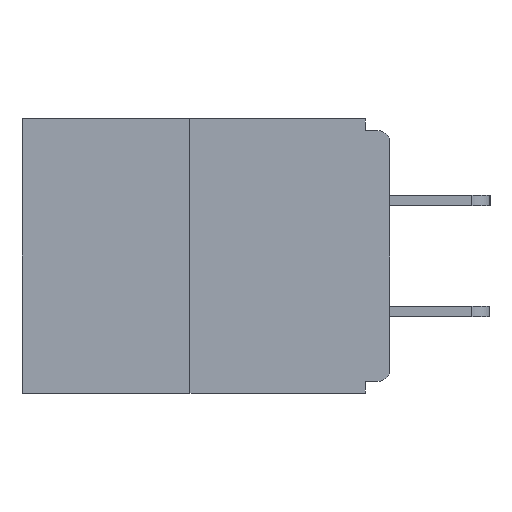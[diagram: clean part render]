
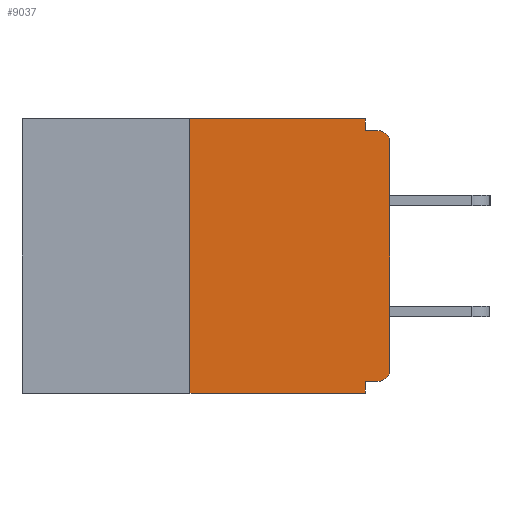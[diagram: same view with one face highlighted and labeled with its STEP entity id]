
A CAD part, left-side view. The second image highlights one B-rep face of the part: STEP entity #9037.
In plain terms, the highlighted planar face has unit normal (-1, 0, 0).
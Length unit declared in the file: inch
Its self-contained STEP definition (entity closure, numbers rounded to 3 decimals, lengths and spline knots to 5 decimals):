
#4 = ORIENTED_EDGE ( 'NONE', *, *, #11150, .F. ) ;
#123 = EDGE_LOOP ( 'NONE', ( #939, #2051, #2293, #3961, #8001, #12111, #1649, #12797, #4116, #4 ) ) ;
#710 = VERTEX_POINT ( 'NONE', #12947 ) ;
#714 = CARTESIAN_POINT ( 'NONE',  ( 0., 0., -0.313 ) ) ;
#939 = ORIENTED_EDGE ( 'NONE', *, *, #2842, .F. ) ;
#1029 = CARTESIAN_POINT ( 'NONE',  ( 0., 0.46, 0. ) ) ;
#1086 = VECTOR ( 'NONE', #10033, 39.37008 ) ;
#1126 = CARTESIAN_POINT ( 'NONE',  ( 0., 0., -0.015 ) ) ;
#1252 = AXIS2_PLACEMENT_3D ( 'NONE', #8009, #3715, #13495 ) ;
#1649 = ORIENTED_EDGE ( 'NONE', *, *, #4518, .T. ) ;
#1682 = DIRECTION ( 'NONE',  ( 0., -1., 0. ) ) ;
#2051 = ORIENTED_EDGE ( 'NONE', *, *, #3846, .F. ) ;
#2113 = DIRECTION ( 'NONE',  ( 0., 0., -1. ) ) ;
#2199 = CARTESIAN_POINT ( 'NONE',  ( 0., 0.25, -0.343 ) ) ;
#2293 = ORIENTED_EDGE ( 'NONE', *, *, #7342, .T. ) ;
#2337 = CARTESIAN_POINT ( 'NONE',  ( 0., 0., -0.328 ) ) ;
#2506 = EDGE_CURVE ( 'NONE', #710, #9121, #10953, .T. ) ;
#2724 = DIRECTION ( 'NONE',  ( 0., 0., -1. ) ) ;
#2842 = EDGE_CURVE ( 'NONE', #11272, #7863, #7453, .T. ) ;
#2844 = DIRECTION ( 'NONE',  ( 0., 0., -1. ) ) ;
#3368 = AXIS2_PLACEMENT_3D ( 'NONE', #10597, #12603, #2844 ) ;
#3414 = CARTESIAN_POINT ( 'NONE',  ( 0., 0., 0. ) ) ;
#3503 = CARTESIAN_POINT ( 'NONE',  ( 0., 0.031, -0.328 ) ) ;
#3594 = EDGE_CURVE ( 'NONE', #7146, #11000, #7403, .T. ) ;
#3715 = DIRECTION ( 'NONE',  ( -1., 0., 0. ) ) ;
#3846 = EDGE_CURVE ( 'NONE', #4513, #11272, #9178, .T. ) ;
#3870 = CARTESIAN_POINT ( 'NONE',  ( 0., 0.015, -0.015 ) ) ;
#3961 = ORIENTED_EDGE ( 'NONE', *, *, #8434, .F. ) ;
#4116 = ORIENTED_EDGE ( 'NONE', *, *, #2506, .F. ) ;
#4135 = DIRECTION ( 'NONE',  ( 0., -1., 0. ) ) ;
#4455 = VECTOR ( 'NONE', #14008, 39.37008 ) ;
#4478 = LINE ( 'NONE', #2337, #6018 ) ;
#4513 = VERTEX_POINT ( 'NONE', #2199 ) ;
#4518 = EDGE_CURVE ( 'NONE', #11000, #6006, #5553, .T. ) ;
#4608 = CARTESIAN_POINT ( 'NONE',  ( 0., 0.25, 0. ) ) ;
#5466 = CARTESIAN_POINT ( 'NONE',  ( 0., 0.031, 0. ) ) ;
#5486 = DIRECTION ( 'NONE',  ( 0., 1., 0. ) ) ;
#5553 = LINE ( 'NONE', #3414, #13329 ) ;
#5609 = CARTESIAN_POINT ( 'NONE',  ( 0., 0.015, -0.328 ) ) ;
#5943 = FACE_OUTER_BOUND ( 'NONE', #123, .T. ) ;
#6006 = VERTEX_POINT ( 'NONE', #13749 ) ;
#6018 = VECTOR ( 'NONE', #5486, 39.37008 ) ;
#6039 = CARTESIAN_POINT ( 'NONE',  ( 0., 0.46, -0.343 ) ) ;
#6640 = EDGE_CURVE ( 'NONE', #7146, #8981, #4478, .T. ) ;
#6699 = DIRECTION ( 'NONE',  ( 0., 0., 1. ) ) ;
#7146 = VERTEX_POINT ( 'NONE', #5609 ) ;
#7342 = EDGE_CURVE ( 'NONE', #4513, #10835, #9311, .T. ) ;
#7403 = CIRCLE ( 'NONE', #1252, 0.015 ) ;
#7453 = LINE ( 'NONE', #1029, #4455 ) ;
#7598 = CARTESIAN_POINT ( 'NONE',  ( 0., 0.031, -0.343 ) ) ;
#7863 = VERTEX_POINT ( 'NONE', #12569 ) ;
#8001 = ORIENTED_EDGE ( 'NONE', *, *, #6640, .F. ) ;
#8009 = CARTESIAN_POINT ( 'NONE',  ( 0., 0.015, -0.313 ) ) ;
#8138 = DIRECTION ( 'NONE',  ( 1., 0., 0. ) ) ;
#8434 = EDGE_CURVE ( 'NONE', #8981, #10835, #9732, .T. ) ;
#8981 = VERTEX_POINT ( 'NONE', #3503 ) ;
#9037 = ADVANCED_FACE ( 'NONE', ( #5943 ), #10279, .F. ) ;
#9121 = VERTEX_POINT ( 'NONE', #3870 ) ;
#9178 = LINE ( 'NONE', #4608, #1086 ) ;
#9311 = LINE ( 'NONE', #6039, #13803 ) ;
#9528 = CIRCLE ( 'NONE', #3368, 0.015 ) ;
#9560 = EDGE_CURVE ( 'NONE', #6006, #9121, #9528, .T. ) ;
#9732 = LINE ( 'NONE', #7598, #12444 ) ;
#10033 = DIRECTION ( 'NONE',  ( 0., 0., 1. ) ) ;
#10279 = PLANE ( 'NONE',  #11314 ) ;
#10314 = CARTESIAN_POINT ( 'NONE',  ( 0., 0.031, -0.343 ) ) ;
#10597 = CARTESIAN_POINT ( 'NONE',  ( 0., 0.015, -0.03 ) ) ;
#10835 = VERTEX_POINT ( 'NONE', #10314 ) ;
#10953 = LINE ( 'NONE', #1126, #12747 ) ;
#11000 = VERTEX_POINT ( 'NONE', #714 ) ;
#11150 = EDGE_CURVE ( 'NONE', #7863, #710, #11879, .T. ) ;
#11201 = CARTESIAN_POINT ( 'NONE',  ( 0., 0.25, 0. ) ) ;
#11272 = VERTEX_POINT ( 'NONE', #11201 ) ;
#11314 = AXIS2_PLACEMENT_3D ( 'NONE', #13555, #8138, #2724 ) ;
#11879 = LINE ( 'NONE', #5466, #12892 ) ;
#11936 = DIRECTION ( 'NONE',  ( 0., 0., -1. ) ) ;
#12111 = ORIENTED_EDGE ( 'NONE', *, *, #3594, .T. ) ;
#12444 = VECTOR ( 'NONE', #11936, 39.37008 ) ;
#12569 = CARTESIAN_POINT ( 'NONE',  ( 0., 0.031, 0. ) ) ;
#12603 = DIRECTION ( 'NONE',  ( -1., 0., 0. ) ) ;
#12747 = VECTOR ( 'NONE', #4135, 39.37008 ) ;
#12797 = ORIENTED_EDGE ( 'NONE', *, *, #9560, .T. ) ;
#12892 = VECTOR ( 'NONE', #2113, 39.37008 ) ;
#12947 = CARTESIAN_POINT ( 'NONE',  ( 0., 0.031, -0.015 ) ) ;
#13329 = VECTOR ( 'NONE', #6699, 39.37008 ) ;
#13495 = DIRECTION ( 'NONE',  ( 0., 0., -1. ) ) ;
#13555 = CARTESIAN_POINT ( 'NONE',  ( 0., 0.46, 0. ) ) ;
#13749 = CARTESIAN_POINT ( 'NONE',  ( 0., 0., -0.03 ) ) ;
#13803 = VECTOR ( 'NONE', #1682, 39.37008 ) ;
#14008 = DIRECTION ( 'NONE',  ( 0., -1., 0. ) ) ;
